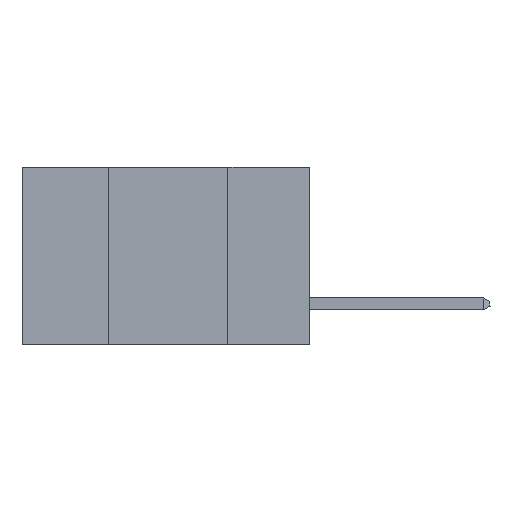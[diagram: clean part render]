
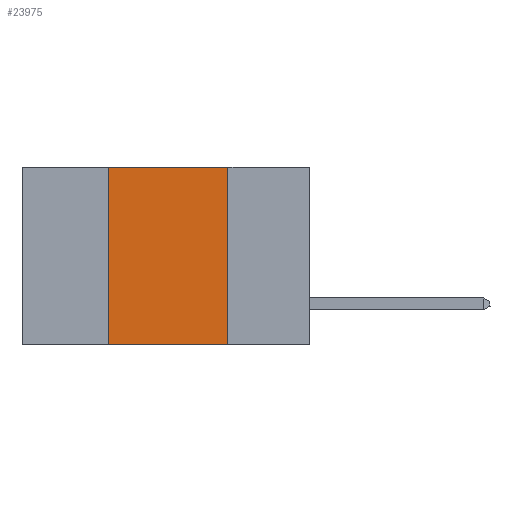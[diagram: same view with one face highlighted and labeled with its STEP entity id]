
A CAD part, left-side view. The second image highlights one B-rep face of the part: STEP entity #23975.
In plain terms, the highlighted planar face has unit normal (-1, 0, 0).
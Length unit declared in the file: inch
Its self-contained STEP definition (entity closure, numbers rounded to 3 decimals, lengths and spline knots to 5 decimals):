
#67 = ORIENTED_EDGE ( 'NONE', *, *, #5861, .F. ) ;
#1181 = CARTESIAN_POINT ( 'NONE',  ( 0., 0.6, 0. ) ) ;
#1204 = VERTEX_POINT ( 'NONE', #1650 ) ;
#1650 = CARTESIAN_POINT ( 'NONE',  ( 0., 0.42, -0.37 ) ) ;
#2108 = EDGE_LOOP ( 'NONE', ( #67, #9687, #7049, #24795 ) ) ;
#4021 = VECTOR ( 'NONE', #5063, 39.37008 ) ;
#4183 = FACE_OUTER_BOUND ( 'NONE', #2108, .T. ) ;
#4909 = CARTESIAN_POINT ( 'NONE',  ( 0., 0.42, 0. ) ) ;
#5063 = DIRECTION ( 'NONE',  ( 0., -1., 0. ) ) ;
#5861 = EDGE_CURVE ( 'NONE', #8700, #11223, #25235, .T. ) ;
#7049 = ORIENTED_EDGE ( 'NONE', *, *, #20914, .F. ) ;
#7816 = VECTOR ( 'NONE', #24855, 39.37008 ) ;
#7983 = EDGE_CURVE ( 'NONE', #25952, #8700, #14603, .T. ) ;
#8184 = LINE ( 'NONE', #20873, #7816 ) ;
#8700 = VERTEX_POINT ( 'NONE', #11410 ) ;
#9687 = ORIENTED_EDGE ( 'NONE', *, *, #7983, .F. ) ;
#10184 = EDGE_CURVE ( 'NONE', #1204, #11223, #8184, .T. ) ;
#10784 = CARTESIAN_POINT ( 'NONE',  ( 0., 0.17, 0. ) ) ;
#11223 = VERTEX_POINT ( 'NONE', #17898 ) ;
#11410 = CARTESIAN_POINT ( 'NONE',  ( 0., 0.17, 0. ) ) ;
#14603 = LINE ( 'NONE', #17939, #4021 ) ;
#14787 = DIRECTION ( 'NONE',  ( 0., 0., -1. ) ) ;
#17898 = CARTESIAN_POINT ( 'NONE',  ( 0., 0.17, -0.37 ) ) ;
#17939 = CARTESIAN_POINT ( 'NONE',  ( 0., 0.6, 0. ) ) ;
#18298 = VECTOR ( 'NONE', #14787, 39.37008 ) ;
#20294 = DIRECTION ( 'NONE',  ( 0., 0., -1. ) ) ;
#20873 = CARTESIAN_POINT ( 'NONE',  ( 0., 0.6, -0.37 ) ) ;
#20914 = EDGE_CURVE ( 'NONE', #1204, #25952, #22179, .T. ) ;
#22179 = LINE ( 'NONE', #22317, #24171 ) ;
#22317 = CARTESIAN_POINT ( 'NONE',  ( 0., 0.42, 0. ) ) ;
#22958 = AXIS2_PLACEMENT_3D ( 'NONE', #1181, #26047, #20294 ) ;
#23975 = ADVANCED_FACE ( 'NONE', ( #4183 ), #26609, .F. ) ;
#24171 = VECTOR ( 'NONE', #26593, 39.37008 ) ;
#24795 = ORIENTED_EDGE ( 'NONE', *, *, #10184, .T. ) ;
#24855 = DIRECTION ( 'NONE',  ( 0., -1., 0. ) ) ;
#25235 = LINE ( 'NONE', #10784, #18298 ) ;
#25952 = VERTEX_POINT ( 'NONE', #4909 ) ;
#26047 = DIRECTION ( 'NONE',  ( 1., 0., 0. ) ) ;
#26593 = DIRECTION ( 'NONE',  ( 0., 0., 1. ) ) ;
#26609 = PLANE ( 'NONE',  #22958 ) ;
